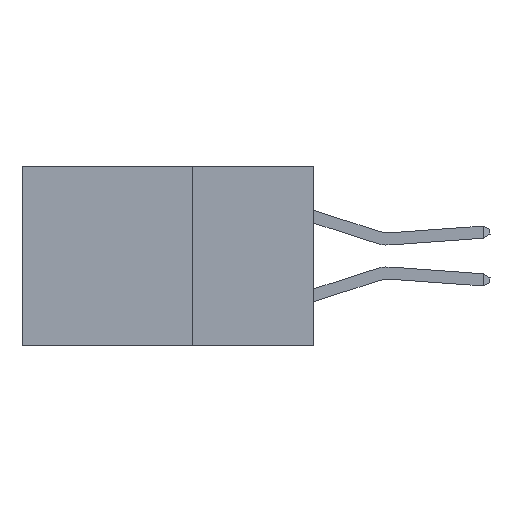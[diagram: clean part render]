
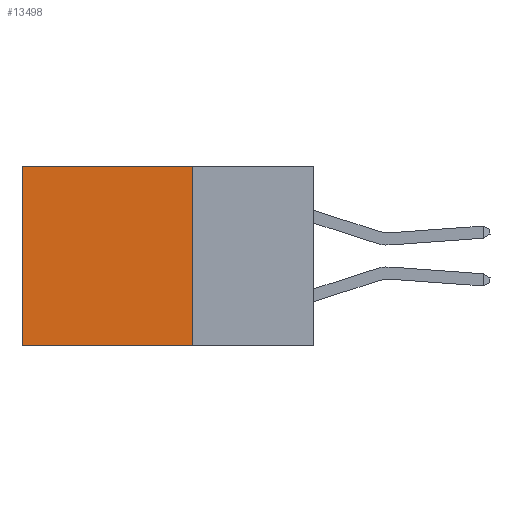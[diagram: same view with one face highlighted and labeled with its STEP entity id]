
A CAD part, left-side view. The second image highlights one B-rep face of the part: STEP entity #13498.
In plain terms, the highlighted planar face has unit normal (-1, 0, 0).
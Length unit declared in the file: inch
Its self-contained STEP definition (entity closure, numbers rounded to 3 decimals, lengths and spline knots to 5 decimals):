
#1747 = LINE ( 'NONE', #4855, #15316 ) ;
#1764 = VECTOR ( 'NONE', #20768, 39.37008 ) ;
#2281 = AXIS2_PLACEMENT_3D ( 'NONE', #23838, #15272, #7390 ) ;
#2368 = VECTOR ( 'NONE', #33061, 39.37008 ) ;
#3422 = LINE ( 'NONE', #9436, #1764 ) ;
#3475 = ORIENTED_EDGE ( 'NONE', *, *, #32139, .T. ) ;
#4570 = EDGE_CURVE ( 'NONE', #13168, #21549, #1747, .T. ) ;
#4855 = CARTESIAN_POINT ( 'NONE',  ( 0.2875, 0.25, -0.37 ) ) ;
#7315 = ORIENTED_EDGE ( 'NONE', *, *, #14594, .F. ) ;
#7390 = DIRECTION ( 'NONE',  ( 0., 0., -1. ) ) ;
#8341 = CARTESIAN_POINT ( 'NONE',  ( 0.2875, 0.6, 0. ) ) ;
#8508 = CARTESIAN_POINT ( 'NONE',  ( 0.2875, 0.25, 0. ) ) ;
#9436 = CARTESIAN_POINT ( 'NONE',  ( 0.2875, 0.25, 0. ) ) ;
#10696 = DIRECTION ( 'NONE',  ( 0., 1., 0. ) ) ;
#13168 = VERTEX_POINT ( 'NONE', #25330 ) ;
#13498 = ADVANCED_FACE ( 'NONE', ( #32243 ), #34983, .F. ) ;
#14594 = EDGE_CURVE ( 'NONE', #21718, #13168, #3422, .T. ) ;
#14874 = CARTESIAN_POINT ( 'NONE',  ( 0.2875, 0.6, -0.37 ) ) ;
#15272 = DIRECTION ( 'NONE',  ( 1., 0., 0. ) ) ;
#15316 = VECTOR ( 'NONE', #10696, 39.37008 ) ;
#16322 = EDGE_CURVE ( 'NONE', #20511, #21549, #33355, .T. ) ;
#17422 = ORIENTED_EDGE ( 'NONE', *, *, #4570, .F. ) ;
#20511 = VERTEX_POINT ( 'NONE', #22124 ) ;
#20768 = DIRECTION ( 'NONE',  ( 0., 0., -1. ) ) ;
#21549 = VERTEX_POINT ( 'NONE', #14874 ) ;
#21718 = VERTEX_POINT ( 'NONE', #26360 ) ;
#22124 = CARTESIAN_POINT ( 'NONE',  ( 0.2875, 0.6, 0. ) ) ;
#23838 = CARTESIAN_POINT ( 'NONE',  ( 0.2875, 0.25, 0. ) ) ;
#23867 = ORIENTED_EDGE ( 'NONE', *, *, #16322, .T. ) ;
#24389 = EDGE_LOOP ( 'NONE', ( #23867, #17422, #7315, #3475 ) ) ;
#25330 = CARTESIAN_POINT ( 'NONE',  ( 0.2875, 0.25, -0.37 ) ) ;
#26360 = CARTESIAN_POINT ( 'NONE',  ( 0.2875, 0.25, 0. ) ) ;
#32139 = EDGE_CURVE ( 'NONE', #21718, #20511, #33337, .T. ) ;
#32243 = FACE_OUTER_BOUND ( 'NONE', #24389, .T. ) ;
#33061 = DIRECTION ( 'NONE',  ( 0., 1., 0. ) ) ;
#33325 = VECTOR ( 'NONE', #33542, 39.37008 ) ;
#33337 = LINE ( 'NONE', #8508, #2368 ) ;
#33355 = LINE ( 'NONE', #8341, #33325 ) ;
#33542 = DIRECTION ( 'NONE',  ( 0., 0., -1. ) ) ;
#34983 = PLANE ( 'NONE',  #2281 ) ;
